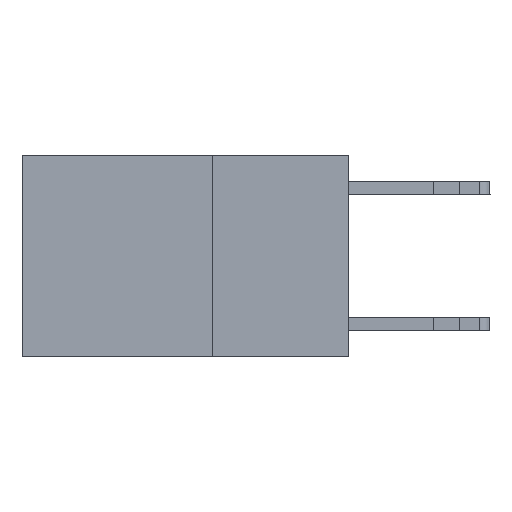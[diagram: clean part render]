
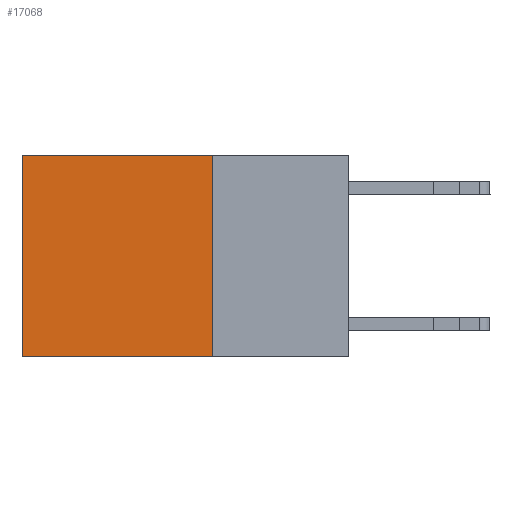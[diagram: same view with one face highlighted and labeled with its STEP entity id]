
A CAD part, left-side view. The second image highlights one B-rep face of the part: STEP entity #17068.
In plain terms, the highlighted planar face has unit normal (-1, 0, 0).
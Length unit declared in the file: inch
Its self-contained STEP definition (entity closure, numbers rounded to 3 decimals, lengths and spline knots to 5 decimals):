
#185 = ORIENTED_EDGE ( 'NONE', *, *, #12521, .F. ) ;
#549 = DIRECTION ( 'NONE',  ( 1., 0., 0. ) ) ;
#734 = CARTESIAN_POINT ( 'NONE',  ( 0.2625, 0.6, 0. ) ) ;
#1063 = EDGE_LOOP ( 'NONE', ( #19845, #185, #7547, #16825 ) ) ;
#1517 = CARTESIAN_POINT ( 'NONE',  ( 0.2625, 0.25, -0.37 ) ) ;
#1709 = LINE ( 'NONE', #11187, #7083 ) ;
#3667 = CARTESIAN_POINT ( 'NONE',  ( 0.2625, 0.25, 0. ) ) ;
#4932 = DIRECTION ( 'NONE',  ( 0., 1., 0. ) ) ;
#4951 = LINE ( 'NONE', #1517, #7924 ) ;
#5324 = PLANE ( 'NONE',  #8178 ) ;
#5424 = EDGE_CURVE ( 'NONE', #16775, #9116, #7881, .T. ) ;
#6329 = CARTESIAN_POINT ( 'NONE',  ( 0.2625, 0.25, 0. ) ) ;
#6707 = EDGE_CURVE ( 'NONE', #9275, #16352, #6768, .T. ) ;
#6768 = LINE ( 'NONE', #734, #14587 ) ;
#7083 = VECTOR ( 'NONE', #4932, 39.37008 ) ;
#7547 = ORIENTED_EDGE ( 'NONE', *, *, #5424, .F. ) ;
#7851 = EDGE_CURVE ( 'NONE', #16775, #9275, #1709, .T. ) ;
#7881 = LINE ( 'NONE', #6329, #14037 ) ;
#7924 = VECTOR ( 'NONE', #9726, 39.37008 ) ;
#8178 = AXIS2_PLACEMENT_3D ( 'NONE', #10004, #549, #16403 ) ;
#9116 = VERTEX_POINT ( 'NONE', #11547 ) ;
#9275 = VERTEX_POINT ( 'NONE', #20464 ) ;
#9726 = DIRECTION ( 'NONE',  ( 0., 1., 0. ) ) ;
#10004 = CARTESIAN_POINT ( 'NONE',  ( 0.2625, 0.25, 0. ) ) ;
#11187 = CARTESIAN_POINT ( 'NONE',  ( 0.2625, 0.25, 0. ) ) ;
#11547 = CARTESIAN_POINT ( 'NONE',  ( 0.2625, 0.25, -0.37 ) ) ;
#12521 = EDGE_CURVE ( 'NONE', #9116, #16352, #4951, .T. ) ;
#12700 = DIRECTION ( 'NONE',  ( 0., 0., -1. ) ) ;
#14037 = VECTOR ( 'NONE', #12700, 39.37008 ) ;
#14587 = VECTOR ( 'NONE', #14697, 39.37008 ) ;
#14697 = DIRECTION ( 'NONE',  ( 0., 0., -1. ) ) ;
#14824 = FACE_OUTER_BOUND ( 'NONE', #1063, .T. ) ;
#16352 = VERTEX_POINT ( 'NONE', #19654 ) ;
#16403 = DIRECTION ( 'NONE',  ( 0., 0., -1. ) ) ;
#16775 = VERTEX_POINT ( 'NONE', #3667 ) ;
#16825 = ORIENTED_EDGE ( 'NONE', *, *, #7851, .T. ) ;
#17068 = ADVANCED_FACE ( 'NONE', ( #14824 ), #5324, .F. ) ;
#19654 = CARTESIAN_POINT ( 'NONE',  ( 0.2625, 0.6, -0.37 ) ) ;
#19845 = ORIENTED_EDGE ( 'NONE', *, *, #6707, .T. ) ;
#20464 = CARTESIAN_POINT ( 'NONE',  ( 0.2625, 0.6, 0. ) ) ;
